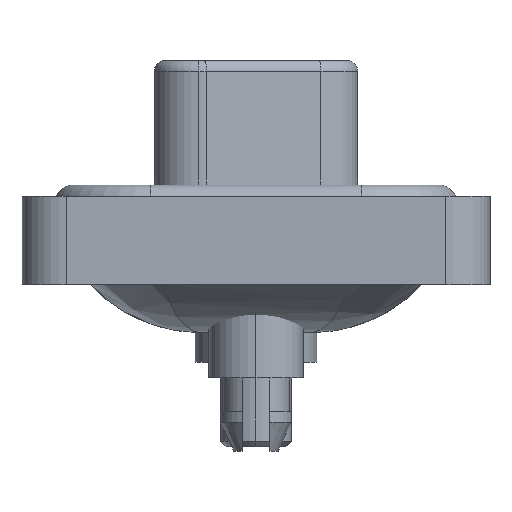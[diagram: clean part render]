
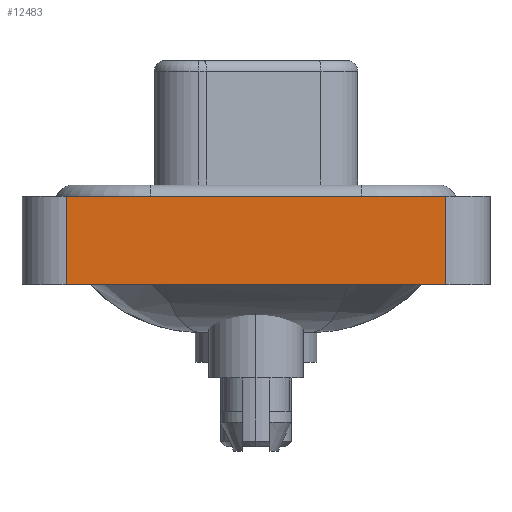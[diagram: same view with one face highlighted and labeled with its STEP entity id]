
A CAD part, left-side view. The second image highlights one B-rep face of the part: STEP entity #12483.
In plain terms, the highlighted planar face has unit normal (-1, 0, 0).
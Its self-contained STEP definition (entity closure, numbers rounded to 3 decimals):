
#1597 = ORIENTED_EDGE ( 'NONE', *, *, #18611, .F. ) ;
#2164 = DIRECTION ( 'NONE',  ( 0., 0., 1. ) ) ;
#2248 = CARTESIAN_POINT ( 'NONE',  ( -7.25, -8.55, -3.6 ) ) ;
#3340 = VECTOR ( 'NONE', #2164, 1000. ) ;
#3440 = CARTESIAN_POINT ( 'NONE',  ( -7.25, 8.55, 0.4 ) ) ;
#4104 = DIRECTION ( 'NONE',  ( -1., 0., 0. ) ) ;
#4123 = VERTEX_POINT ( 'NONE', #3440 ) ;
#4238 = ORIENTED_EDGE ( 'NONE', *, *, #7005, .F. ) ;
#4993 = DIRECTION ( 'NONE',  ( 0., -1., 0. ) ) ;
#5819 = CARTESIAN_POINT ( 'NONE',  ( -7.25, -8.55, 0.4 ) ) ;
#5841 = FACE_OUTER_BOUND ( 'NONE', #10399, .T. ) ;
#6627 = LINE ( 'NONE', #2248, #16175 ) ;
#7005 = EDGE_CURVE ( 'NONE', #18185, #4123, #8260, .T. ) ;
#7463 = DIRECTION ( 'NONE',  ( 0., 0., 1. ) ) ;
#8260 = LINE ( 'NONE', #11399, #3340 ) ;
#8653 = VECTOR ( 'NONE', #18191, 1000. ) ;
#10399 = EDGE_LOOP ( 'NONE', ( #11675, #1597, #4238, #12718 ) ) ;
#10687 = EDGE_CURVE ( 'NONE', #15095, #18055, #16548, .T. ) ;
#11399 = CARTESIAN_POINT ( 'NONE',  ( -7.25, 8.55, -3.6 ) ) ;
#11675 = ORIENTED_EDGE ( 'NONE', *, *, #10687, .T. ) ;
#11819 = PLANE ( 'NONE',  #12941 ) ;
#12180 = CARTESIAN_POINT ( 'NONE',  ( -7.25, -8.55, -3.6 ) ) ;
#12483 = ADVANCED_FACE ( 'NONE', ( #5841 ), #11819, .T. ) ;
#12713 = EDGE_CURVE ( 'NONE', #18185, #15095, #6627, .T. ) ;
#12718 = ORIENTED_EDGE ( 'NONE', *, *, #12713, .T. ) ;
#12909 = CARTESIAN_POINT ( 'NONE',  ( -7.25, 8.55, -3.6 ) ) ;
#12941 = AXIS2_PLACEMENT_3D ( 'NONE', #18010, #4104, #7463 ) ;
#14800 = CARTESIAN_POINT ( 'NONE',  ( -7.25, -8.55, -3.6 ) ) ;
#15095 = VERTEX_POINT ( 'NONE', #14800 ) ;
#15943 = VECTOR ( 'NONE', #19486, 1000. ) ;
#16175 = VECTOR ( 'NONE', #4993, 1000. ) ;
#16548 = LINE ( 'NONE', #12180, #15943 ) ;
#17587 = CARTESIAN_POINT ( 'NONE',  ( -7.25, -8.55, 0.4 ) ) ;
#18010 = CARTESIAN_POINT ( 'NONE',  ( -7.25, -8.55, -3.6 ) ) ;
#18055 = VERTEX_POINT ( 'NONE', #17587 ) ;
#18185 = VERTEX_POINT ( 'NONE', #12909 ) ;
#18191 = DIRECTION ( 'NONE',  ( 0., -1., 0. ) ) ;
#18611 = EDGE_CURVE ( 'NONE', #4123, #18055, #19720, .T. ) ;
#19486 = DIRECTION ( 'NONE',  ( 0., 0., 1. ) ) ;
#19720 = LINE ( 'NONE', #5819, #8653 ) ;
